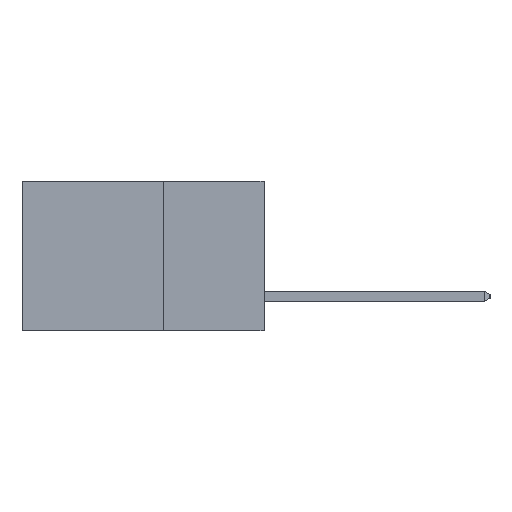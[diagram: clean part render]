
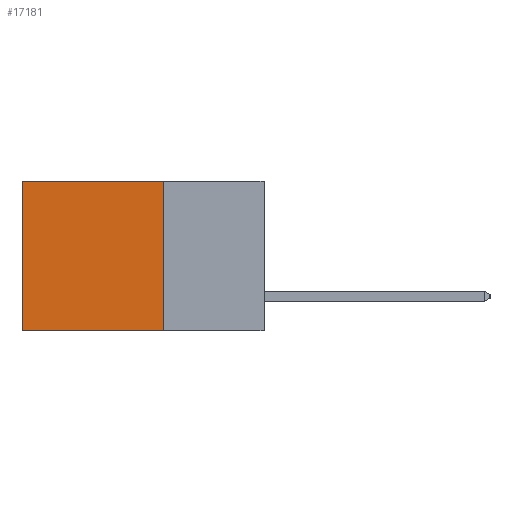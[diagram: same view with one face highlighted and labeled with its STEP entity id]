
A CAD part, left-side view. The second image highlights one B-rep face of the part: STEP entity #17181.
In plain terms, the highlighted planar face has unit normal (-1, 0, 0).
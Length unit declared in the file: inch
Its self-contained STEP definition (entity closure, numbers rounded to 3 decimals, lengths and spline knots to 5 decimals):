
#106 = LINE ( 'NONE', #9795, #14102 ) ;
#2101 = EDGE_LOOP ( 'NONE', ( #10479, #13939, #2764, #6639 ) ) ;
#2427 = LINE ( 'NONE', #5741, #16325 ) ;
#2764 = ORIENTED_EDGE ( 'NONE', *, *, #12858, .F. ) ;
#3177 = VERTEX_POINT ( 'NONE', #17052 ) ;
#3515 = FACE_OUTER_BOUND ( 'NONE', #2101, .T. ) ;
#4643 = EDGE_CURVE ( 'NONE', #3177, #8069, #2427, .T. ) ;
#4720 = VERTEX_POINT ( 'NONE', #4923 ) ;
#4923 = CARTESIAN_POINT ( 'NONE',  ( 0.2615, 0.25, -0.37 ) ) ;
#4924 = DIRECTION ( 'NONE',  ( 1., 0., 0. ) ) ;
#5096 = DIRECTION ( 'NONE',  ( 0., 1., 0. ) ) ;
#5672 = DIRECTION ( 'NONE',  ( 0., 0., -1. ) ) ;
#5741 = CARTESIAN_POINT ( 'NONE',  ( 0.2615, 0.6, -0.37 ) ) ;
#6639 = ORIENTED_EDGE ( 'NONE', *, *, #7041, .T. ) ;
#6829 = VECTOR ( 'NONE', #5096, 39.37008 ) ;
#7041 = EDGE_CURVE ( 'NONE', #10992, #3177, #9774, .T. ) ;
#7828 = CARTESIAN_POINT ( 'NONE',  ( 0.2615, 0.25, 0. ) ) ;
#7872 = DIRECTION ( 'NONE',  ( 0., 1., 0. ) ) ;
#8069 = VERTEX_POINT ( 'NONE', #16632 ) ;
#8971 = CARTESIAN_POINT ( 'NONE',  ( 0.2615, 0.25, -0.37 ) ) ;
#9774 = LINE ( 'NONE', #7828, #16441 ) ;
#9795 = CARTESIAN_POINT ( 'NONE',  ( 0.2615, 0.25, -0.37 ) ) ;
#10479 = ORIENTED_EDGE ( 'NONE', *, *, #4643, .T. ) ;
#10992 = VERTEX_POINT ( 'NONE', #12709 ) ;
#11848 = EDGE_CURVE ( 'NONE', #4720, #8069, #13934, .T. ) ;
#12709 = CARTESIAN_POINT ( 'NONE',  ( 0.2615, 0.25, 0. ) ) ;
#12858 = EDGE_CURVE ( 'NONE', #10992, #4720, #106, .T. ) ;
#13088 = CARTESIAN_POINT ( 'NONE',  ( 0.2615, 0.25, -0.37 ) ) ;
#13934 = LINE ( 'NONE', #13088, #6829 ) ;
#13939 = ORIENTED_EDGE ( 'NONE', *, *, #11848, .F. ) ;
#14102 = VECTOR ( 'NONE', #16485, 39.37008 ) ;
#14333 = DIRECTION ( 'NONE',  ( 0., 0., -1. ) ) ;
#15611 = PLANE ( 'NONE',  #17265 ) ;
#16325 = VECTOR ( 'NONE', #5672, 39.37008 ) ;
#16441 = VECTOR ( 'NONE', #7872, 39.37008 ) ;
#16485 = DIRECTION ( 'NONE',  ( 0., 0., -1. ) ) ;
#16632 = CARTESIAN_POINT ( 'NONE',  ( 0.2615, 0.6, -0.37 ) ) ;
#17052 = CARTESIAN_POINT ( 'NONE',  ( 0.2615, 0.6, 0. ) ) ;
#17181 = ADVANCED_FACE ( 'NONE', ( #3515 ), #15611, .F. ) ;
#17265 = AXIS2_PLACEMENT_3D ( 'NONE', #8971, #4924, #14333 ) ;
